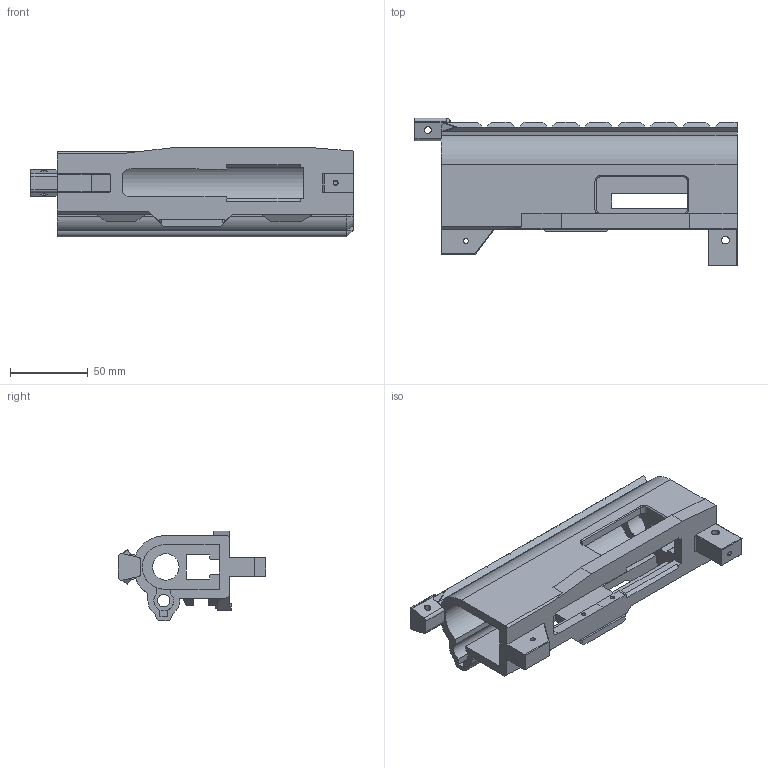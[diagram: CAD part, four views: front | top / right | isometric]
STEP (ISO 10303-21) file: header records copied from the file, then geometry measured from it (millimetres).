
FILE_DESCRIPTION(('STEP AP214'),'1');
FILE_NAME('MOD9_upper_receiver editable solid.stp','2020-07-27T18:43:48',(' '),(' '),'Spatial InterOp 3D',' ',' ');
FILE_SCHEMA(('AUTOMOTIVE_DESIGN { 1 0 10303 214 1 1 1 1 }'));
Length unit declared in the file: metre
Products named in the file (1): Solid
Bounding box: 207.36 x 94.9 x 57.79 mm (x, y, z)
Volume: 248938.8 mm3; surface area: 84239.1 mm2
Topology: 1 solids, 1 shells, 277 faces, 753 edges, 478 vertices
Faces by surface type: plane 197, cylinder 54, cone 18, torus 4, bspline 4
Entity records: 8858 total; most frequent: CARTESIAN_POINT 1787, ORIENTED_EDGE 1502, DIRECTION 1405, EDGE_CURVE 751, LINE 589, VECTOR 589, VERTEX_POINT 478, AXIS2_PLACEMENT_3D 408
